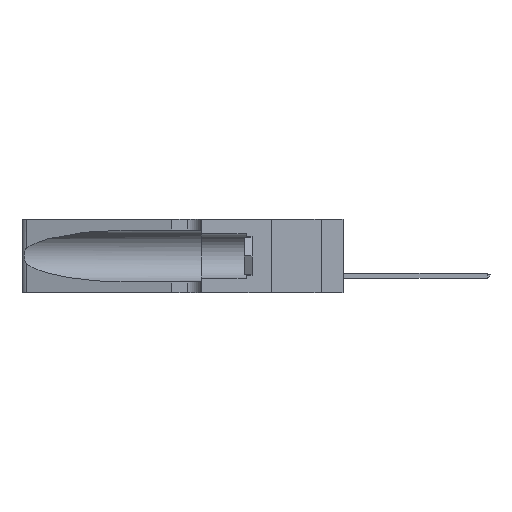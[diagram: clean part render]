
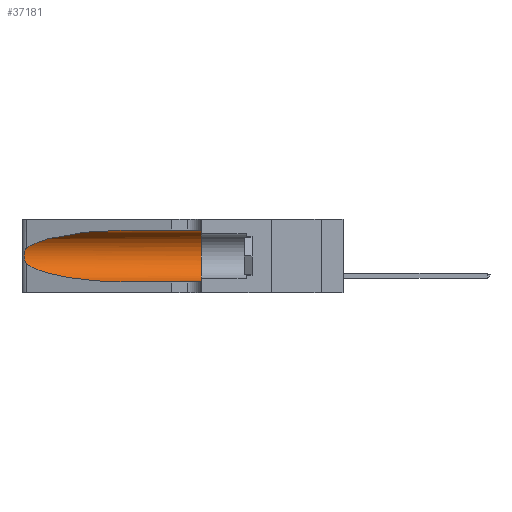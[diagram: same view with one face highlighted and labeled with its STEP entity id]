
A CAD part, left-side view. The second image highlights one B-rep face of the part: STEP entity #37181.
In plain terms, the highlighted cylindrical face has radius 3.308 mm (diameter 6.617 mm), a partial arc.
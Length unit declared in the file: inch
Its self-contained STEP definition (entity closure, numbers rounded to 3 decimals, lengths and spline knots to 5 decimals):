
#881 = CARTESIAN_POINT ( 'NONE',  ( 0.25487, 1.22718, 0.14631 ) ) ;
#1466 = CARTESIAN_POINT ( 'NONE',  ( 0.1305, 0.72297, 0.05475 ) ) ;
#2093 = CARTESIAN_POINT ( 'NONE',  ( 0.25787, 1.23484, 0.2124 ) ) ;
#2144 = CARTESIAN_POINT ( 'NONE',  ( 0.1305, 0.72297, 0.05475 ) ) ;
#2491 = CARTESIAN_POINT ( 'NONE',  ( 0.25487, 1.22718, 0.22369 ) ) ;
#3754 = EDGE_LOOP ( 'NONE', ( #43266, #40965, #35570, #26152, #20434, #30352 ) ) ;
#4437 = CARTESIAN_POINT ( 'NONE',  ( 0.1305, 0.35, 0.05475 ) ) ;
#4851 = CARTESIAN_POINT ( 'NONE',  ( 0.18966, 0.96281, 0.05475 ) ) ;
#5200 = CARTESIAN_POINT ( 'NONE',  ( 0.1305, 0.35, 0.185 ) ) ;
#5901 = CARTESIAN_POINT ( 'NONE',  ( 0.25789, 1.23486, 0.15765 ) ) ;
#6373 = VECTOR ( 'NONE', #9385, 39.37008 ) ;
#8772 = CARTESIAN_POINT ( 'NONE',  ( 0.1305, 0.72297, 0.31525 ) ) ;
#9170 = CARTESIAN_POINT ( 'NONE',  ( 0.2373, 1.15595, 0.28018 ) ) ;
#9385 = DIRECTION ( 'NONE',  ( 0., -1., 0. ) ) ;
#9574 = VERTEX_POINT ( 'NONE', #4437 ) ;
#9578 = CARTESIAN_POINT ( 'NONE',  ( 0.26017, 1.23833, 0.17102 ) ) ;
#10014 = FACE_OUTER_BOUND ( 'NONE', #3754, .T. ) ;
#10822 = AXIS2_PLACEMENT_3D ( 'NONE', #30652, #23936, #27171 ) ;
#11072 = CYLINDRICAL_SURFACE ( 'NONE', #10822, 0.13025 ) ;
#11306 = EDGE_CURVE ( 'NONE', #39586, #36020, #29764, .T. ) ;
#11681 = CARTESIAN_POINT ( 'NONE',  ( 0.1305, 1.61858, 0.31525 ) ) ;
#11821 = EDGE_CURVE ( 'NONE', #34026, #34625, #21637, .T. ) ;
#11862 = CARTESIAN_POINT ( 'NONE',  ( 0.2373, 1.15595, 0.08982 ) ) ;
#12467 = CARTESIAN_POINT ( 'NONE',  ( 0.25487, 1.22718, 0.22369 ) ) ;
#12657 = CARTESIAN_POINT ( 'NONE',  ( 0.1305, 0.72297, 0.31525 ) ) ;
#12757 = CARTESIAN_POINT ( 'NONE',  ( 0.25854, 1.2359, 0.20912 ) ) ;
#15612 = LINE ( 'NONE', #26387, #6373 ) ;
#18875 = EDGE_CURVE ( 'NONE', #34625, #9574, #15612, .T. ) ;
#19095 = AXIS2_PLACEMENT_3D ( 'NONE', #5200, #39984, #19312 ) ;
#19312 = DIRECTION ( 'NONE',  ( 0., 0., 1. ) ) ;
#19948 = CARTESIAN_POINT ( 'NONE',  ( 0.1305, 0.35, 0.31525 ) ) ;
#20434 = ORIENTED_EDGE ( 'NONE', *, *, #33085, .F. ) ;
#21637 =( BOUNDED_CURVE ( )  B_SPLINE_CURVE ( 3, ( #881, #11862, #4851, #1466 ),
 .UNSPECIFIED., .F., .T. ) 
 B_SPLINE_CURVE_WITH_KNOTS ( ( 4, 4 ),
 ( 3.44316, 4.71239 ),
 .UNSPECIFIED. ) 
 CURVE ( )  GEOMETRIC_REPRESENTATION_ITEM ( )  RATIONAL_B_SPLINE_CURVE ( ( 1., 0.87, 0.87, 1. ) ) 
 REPRESENTATION_ITEM ( '' )  );
#22986 = CIRCLE ( 'NONE', #19095, 0.13025 ) ;
#23660 = LINE ( 'NONE', #11681, #33529 ) ;
#23936 = DIRECTION ( 'NONE',  ( 0., -1., 0. ) ) ;
#26152 = ORIENTED_EDGE ( 'NONE', *, *, #18875, .T. ) ;
#26387 = CARTESIAN_POINT ( 'NONE',  ( 0.1305, 1.61858, 0.05475 ) ) ;
#26728 = CARTESIAN_POINT ( 'NONE',  ( 0.25639, 1.23184, 0.21858 ) ) ;
#27171 = DIRECTION ( 'NONE',  ( 0., 0., -1. ) ) ;
#29721 = DIRECTION ( 'NONE',  ( 0., -1., 0. ) ) ;
#29764 =( BOUNDED_CURVE ( )  B_SPLINE_CURVE ( 3, ( #12657, #29958, #9170, #36992 ),
 .UNSPECIFIED., .F., .F. ) 
 B_SPLINE_CURVE_WITH_KNOTS ( ( 4, 4 ),
 ( 1.5708, 2.84003 ),
 .UNSPECIFIED. ) 
 CURVE ( )  GEOMETRIC_REPRESENTATION_ITEM ( )  RATIONAL_B_SPLINE_CURVE ( ( 1., 0.87, 0.87, 1. ) ) 
 REPRESENTATION_ITEM ( '' )  );
#29958 = CARTESIAN_POINT ( 'NONE',  ( 0.18966, 0.96281, 0.31525 ) ) ;
#30051 = CARTESIAN_POINT ( 'NONE',  ( 0.26018, 1.23835, 0.19895 ) ) ;
#30352 = ORIENTED_EDGE ( 'NONE', *, *, #30599, .F. ) ;
#30599 = EDGE_CURVE ( 'NONE', #39586, #38367, #23660, .T. ) ;
#30652 = CARTESIAN_POINT ( 'NONE',  ( 0.1305, 1.61858, 0.185 ) ) ;
#33085 = EDGE_CURVE ( 'NONE', #38367, #9574, #22986, .T. ) ;
#33438 = CARTESIAN_POINT ( 'NONE',  ( 0.25487, 1.22718, 0.14631 ) ) ;
#33529 = VECTOR ( 'NONE', #29721, 39.37008 ) ;
#33721 = CARTESIAN_POINT ( 'NONE',  ( 0.25555, 1.22993, 0.14849 ) ) ;
#34026 = VERTEX_POINT ( 'NONE', #34448 ) ;
#34448 = CARTESIAN_POINT ( 'NONE',  ( 0.25487, 1.22718, 0.14631 ) ) ;
#34625 = VERTEX_POINT ( 'NONE', #2144 ) ;
#35570 = ORIENTED_EDGE ( 'NONE', *, *, #11821, .T. ) ;
#36020 = VERTEX_POINT ( 'NONE', #2491 ) ;
#36798 = CARTESIAN_POINT ( 'NONE',  ( 0.26075, 1.23896, 0.19203 ) ) ;
#36992 = CARTESIAN_POINT ( 'NONE',  ( 0.25487, 1.22718, 0.22369 ) ) ;
#37020 = EDGE_CURVE ( 'NONE', #36020, #34026, #43959, .T. ) ;
#37181 = ADVANCED_FACE ( 'NONE', ( #10014 ), #11072, .F. ) ;
#37222 = CARTESIAN_POINT ( 'NONE',  ( 0.26075, 1.23896, 0.178 ) ) ;
#37375 = CARTESIAN_POINT ( 'NONE',  ( 0.25639, 1.23186, 0.15144 ) ) ;
#38367 = VERTEX_POINT ( 'NONE', #19948 ) ;
#39586 = VERTEX_POINT ( 'NONE', #8772 ) ;
#39984 = DIRECTION ( 'NONE',  ( 0., 1., 0. ) ) ;
#40835 = CARTESIAN_POINT ( 'NONE',  ( 0.25555, 1.22994, 0.2215 ) ) ;
#40965 = ORIENTED_EDGE ( 'NONE', *, *, #37020, .T. ) ;
#43266 = ORIENTED_EDGE ( 'NONE', *, *, #11306, .T. ) ;
#43872 = CARTESIAN_POINT ( 'NONE',  ( 0.25856, 1.23593, 0.16098 ) ) ;
#43959 = B_SPLINE_CURVE_WITH_KNOTS ( 'NONE', 3,
 ( #12467, #40835, #26728, #2093, #12757, #30051, #36798, #37222, #9578, #43872, #5901, #37375, #33721, #33438 ),
 .UNSPECIFIED., .F., .F.,
 ( 4, 2, 2, 2, 2, 2, 4 ),
 ( 0., 0.00027, 0.00053, 0.00107, 0.0016, 0.00187, 0.00214 ),
 .UNSPECIFIED. ) ;
